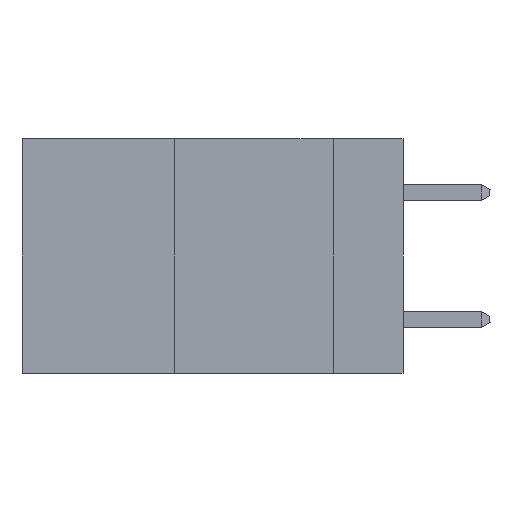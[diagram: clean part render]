
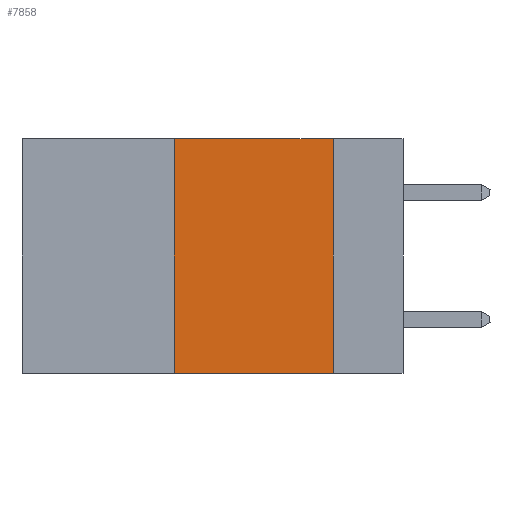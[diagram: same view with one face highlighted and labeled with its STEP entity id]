
A CAD part, left-side view. The second image highlights one B-rep face of the part: STEP entity #7858.
In plain terms, the highlighted planar face has unit normal (-1, 0, 0).
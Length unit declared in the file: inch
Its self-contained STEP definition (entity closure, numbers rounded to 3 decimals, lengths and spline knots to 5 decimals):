
#291 = AXIS2_PLACEMENT_3D ( 'NONE', #19771, #3779, #22447 ) ;
#3779 = DIRECTION ( 'NONE',  ( 1., 0., 0. ) ) ;
#4113 = VECTOR ( 'NONE', #29359, 39.37008 ) ;
#4704 = VERTEX_POINT ( 'NONE', #18223 ) ;
#4998 = LINE ( 'NONE', #27914, #19195 ) ;
#5687 = FACE_OUTER_BOUND ( 'NONE', #28199, .T. ) ;
#6034 = DIRECTION ( 'NONE',  ( 0., -1., 0. ) ) ;
#6845 = DIRECTION ( 'NONE',  ( 0., 0., 1. ) ) ;
#7858 = ADVANCED_FACE ( 'NONE', ( #5687 ), #30328, .F. ) ;
#7971 = ORIENTED_EDGE ( 'NONE', *, *, #32989, .F. ) ;
#10446 = EDGE_CURVE ( 'NONE', #17745, #33269, #25373, .T. ) ;
#17745 = VERTEX_POINT ( 'NONE', #21765 ) ;
#18223 = CARTESIAN_POINT ( 'NONE',  ( 0., 0.36, -0.37 ) ) ;
#18489 = CARTESIAN_POINT ( 'NONE',  ( 0., 0.11, 0. ) ) ;
#19195 = VECTOR ( 'NONE', #30564, 39.37008 ) ;
#19696 = ORIENTED_EDGE ( 'NONE', *, *, #33045, .F. ) ;
#19771 = CARTESIAN_POINT ( 'NONE',  ( 0., 0.6, 0. ) ) ;
#21575 = VECTOR ( 'NONE', #6034, 39.37008 ) ;
#21765 = CARTESIAN_POINT ( 'NONE',  ( 0., 0.36, 0. ) ) ;
#21977 = CARTESIAN_POINT ( 'NONE',  ( 0., 0.6, -0.37 ) ) ;
#22447 = DIRECTION ( 'NONE',  ( 0., 0., -1. ) ) ;
#23749 = VECTOR ( 'NONE', #6845, 39.37008 ) ;
#25373 = LINE ( 'NONE', #26700, #4113 ) ;
#25406 = LINE ( 'NONE', #28131, #23749 ) ;
#26700 = CARTESIAN_POINT ( 'NONE',  ( 0., 0.6, 0. ) ) ;
#27727 = CARTESIAN_POINT ( 'NONE',  ( 0., 0.11, -0.37 ) ) ;
#27822 = LINE ( 'NONE', #21977, #21575 ) ;
#27914 = CARTESIAN_POINT ( 'NONE',  ( 0., 0.11, 0. ) ) ;
#28131 = CARTESIAN_POINT ( 'NONE',  ( 0., 0.36, 0. ) ) ;
#28199 = EDGE_LOOP ( 'NONE', ( #7971, #30884, #19696, #33235 ) ) ;
#28764 = EDGE_CURVE ( 'NONE', #4704, #32209, #27822, .T. ) ;
#29359 = DIRECTION ( 'NONE',  ( 0., -1., 0. ) ) ;
#30328 = PLANE ( 'NONE',  #291 ) ;
#30564 = DIRECTION ( 'NONE',  ( 0., 0., -1. ) ) ;
#30884 = ORIENTED_EDGE ( 'NONE', *, *, #10446, .F. ) ;
#32209 = VERTEX_POINT ( 'NONE', #27727 ) ;
#32989 = EDGE_CURVE ( 'NONE', #33269, #32209, #4998, .T. ) ;
#33045 = EDGE_CURVE ( 'NONE', #4704, #17745, #25406, .T. ) ;
#33235 = ORIENTED_EDGE ( 'NONE', *, *, #28764, .T. ) ;
#33269 = VERTEX_POINT ( 'NONE', #18489 ) ;
